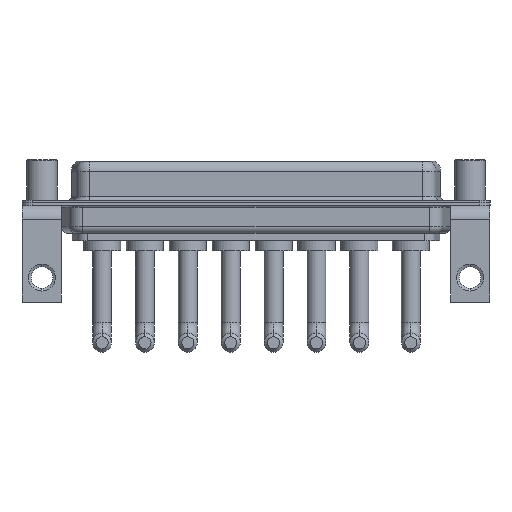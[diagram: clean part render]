
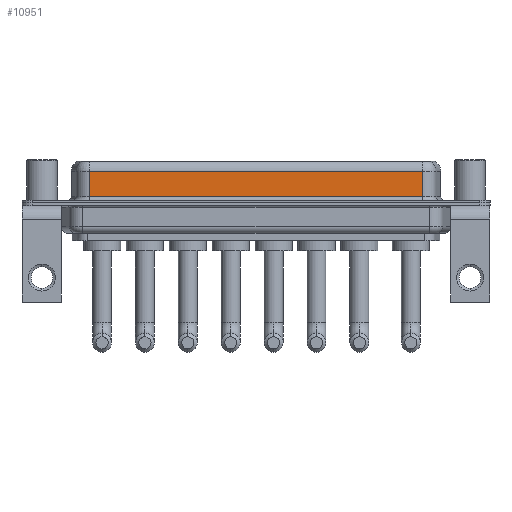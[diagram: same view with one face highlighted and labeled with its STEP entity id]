
A CAD part, front view. The second image highlights one B-rep face of the part: STEP entity #10951.
In plain terms, the highlighted planar face has unit normal (0, -1, 0).
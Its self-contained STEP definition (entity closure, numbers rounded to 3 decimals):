
#243 = DIRECTION ( 'NONE',  ( 0., 1., 0. ) ) ;
#562 = CARTESIAN_POINT ( 'NONE',  ( 7.038, -3.95, 4.65 ) ) ;
#795 = VECTOR ( 'NONE', #5794, 1000. ) ;
#1017 = CARTESIAN_POINT ( 'NONE',  ( 56.462, -3.95, 0.9 ) ) ;
#1355 = VECTOR ( 'NONE', #14061, 1000. ) ;
#1534 = VERTEX_POINT ( 'NONE', #9766 ) ;
#1601 = VERTEX_POINT ( 'NONE', #10168 ) ;
#1747 = EDGE_CURVE ( 'NONE', #1601, #1534, #6257, .T. ) ;
#2382 = EDGE_CURVE ( 'NONE', #12311, #1601, #6591, .T. ) ;
#2966 = VERTEX_POINT ( 'NONE', #9635 ) ;
#3048 = CARTESIAN_POINT ( 'NONE',  ( 7.038, -3.95, 6.4 ) ) ;
#3854 = CARTESIAN_POINT ( 'NONE',  ( 56.462, -3.95, 6.4 ) ) ;
#3931 = FACE_OUTER_BOUND ( 'NONE', #15007, .T. ) ;
#4099 = ORIENTED_EDGE ( 'NONE', *, *, #12032, .F. ) ;
#4194 = VECTOR ( 'NONE', #11442, 1000. ) ;
#4418 = ORIENTED_EDGE ( 'NONE', *, *, #2382, .T. ) ;
#5478 = LINE ( 'NONE', #10510, #795 ) ;
#5794 = DIRECTION ( 'NONE',  ( 0., 0., -1. ) ) ;
#6154 = AXIS2_PLACEMENT_3D ( 'NONE', #3854, #243, #11197 ) ;
#6257 = LINE ( 'NONE', #1017, #1355 ) ;
#6564 = EDGE_CURVE ( 'NONE', #2966, #12311, #15497, .T. ) ;
#6591 = LINE ( 'NONE', #3048, #4194 ) ;
#7536 = PLANE ( 'NONE',  #6154 ) ;
#8406 = DIRECTION ( 'NONE',  ( -1., 0., 0. ) ) ;
#9635 = CARTESIAN_POINT ( 'NONE',  ( 56.462, -3.95, 4.65 ) ) ;
#9766 = CARTESIAN_POINT ( 'NONE',  ( 56.462, -3.95, 0.9 ) ) ;
#10168 = CARTESIAN_POINT ( 'NONE',  ( 7.038, -3.95, 0.9 ) ) ;
#10349 = ORIENTED_EDGE ( 'NONE', *, *, #6564, .T. ) ;
#10510 = CARTESIAN_POINT ( 'NONE',  ( 56.462, -3.95, 6.4 ) ) ;
#10631 = VECTOR ( 'NONE', #8406, 1000. ) ;
#10951 = ADVANCED_FACE ( 'NONE', ( #3931 ), #7536, .F. ) ;
#11197 = DIRECTION ( 'NONE',  ( 0., 0., 1. ) ) ;
#11442 = DIRECTION ( 'NONE',  ( 0., 0., -1. ) ) ;
#12032 = EDGE_CURVE ( 'NONE', #2966, #1534, #5478, .T. ) ;
#12311 = VERTEX_POINT ( 'NONE', #562 ) ;
#14061 = DIRECTION ( 'NONE',  ( 1., 0., 0. ) ) ;
#14444 = CARTESIAN_POINT ( 'NONE',  ( 56.462, -3.95, 4.65 ) ) ;
#14858 = ORIENTED_EDGE ( 'NONE', *, *, #1747, .T. ) ;
#15007 = EDGE_LOOP ( 'NONE', ( #4099, #10349, #4418, #14858 ) ) ;
#15497 = LINE ( 'NONE', #14444, #10631 ) ;
